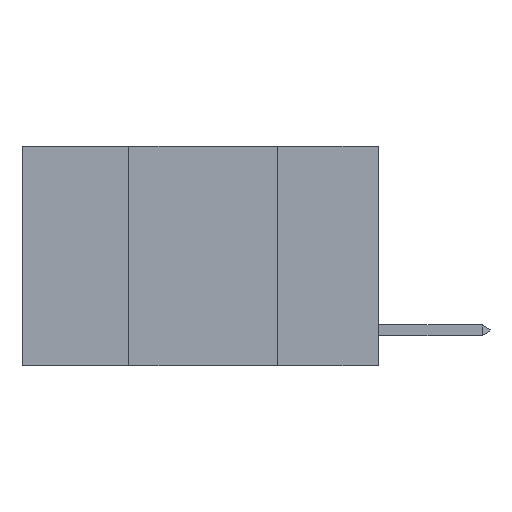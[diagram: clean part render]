
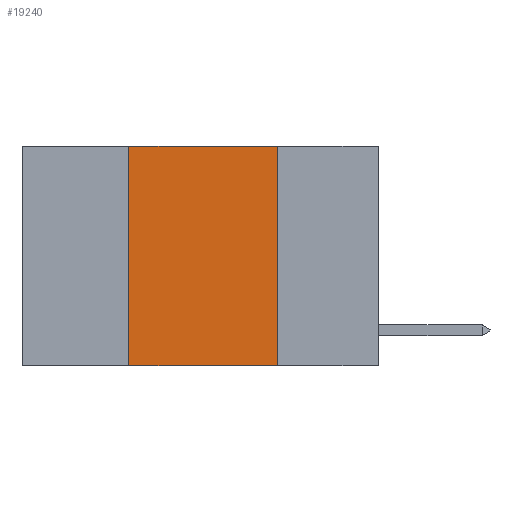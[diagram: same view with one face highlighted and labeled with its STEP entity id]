
A CAD part, left-side view. The second image highlights one B-rep face of the part: STEP entity #19240.
In plain terms, the highlighted planar face has unit normal (-1, 0, 0).
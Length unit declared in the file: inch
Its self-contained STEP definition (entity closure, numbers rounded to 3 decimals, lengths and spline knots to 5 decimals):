
#706 = EDGE_CURVE ( 'NONE', #14869, #10203, #7863, .T. ) ;
#1001 = DIRECTION ( 'NONE',  ( 0., 0., -1. ) ) ;
#1311 = EDGE_CURVE ( 'NONE', #8080, #14869, #18511, .T. ) ;
#1592 = DIRECTION ( 'NONE',  ( 0., -1., 0. ) ) ;
#1633 = FACE_OUTER_BOUND ( 'NONE', #23182, .T. ) ;
#1750 = DIRECTION ( 'NONE',  ( 1., 0., 0. ) ) ;
#4243 = VECTOR ( 'NONE', #1592, 39.37008 ) ;
#5598 = PLANE ( 'NONE',  #17433 ) ;
#6063 = VERTEX_POINT ( 'NONE', #21612 ) ;
#7863 = LINE ( 'NONE', #9908, #4243 ) ;
#8080 = VERTEX_POINT ( 'NONE', #22482 ) ;
#8596 = CARTESIAN_POINT ( 'NONE',  ( 0., 0.42, 0. ) ) ;
#8612 = VECTOR ( 'NONE', #1001, 39.37008 ) ;
#9591 = DIRECTION ( 'NONE',  ( 0., 0., -1. ) ) ;
#9908 = CARTESIAN_POINT ( 'NONE',  ( 0., 0.6, 0. ) ) ;
#10153 = CARTESIAN_POINT ( 'NONE',  ( 0., 0.6, -0.37 ) ) ;
#10203 = VERTEX_POINT ( 'NONE', #22650 ) ;
#10621 = DIRECTION ( 'NONE',  ( 0., 0., 1. ) ) ;
#12024 = ORIENTED_EDGE ( 'NONE', *, *, #1311, .F. ) ;
#12435 = VECTOR ( 'NONE', #22037, 39.37008 ) ;
#13626 = ORIENTED_EDGE ( 'NONE', *, *, #706, .F. ) ;
#14026 = CARTESIAN_POINT ( 'NONE',  ( 0., 0.42, 0. ) ) ;
#14869 = VERTEX_POINT ( 'NONE', #14026 ) ;
#16637 = ORIENTED_EDGE ( 'NONE', *, *, #16826, .T. ) ;
#16826 = EDGE_CURVE ( 'NONE', #8080, #6063, #23457, .T. ) ;
#17433 = AXIS2_PLACEMENT_3D ( 'NONE', #22872, #1750, #9591 ) ;
#18511 = LINE ( 'NONE', #8596, #21848 ) ;
#19240 = ADVANCED_FACE ( 'NONE', ( #1633 ), #5598, .F. ) ;
#20703 = CARTESIAN_POINT ( 'NONE',  ( 0., 0.17, 0. ) ) ;
#21027 = ORIENTED_EDGE ( 'NONE', *, *, #24124, .F. ) ;
#21612 = CARTESIAN_POINT ( 'NONE',  ( 0., 0.17, -0.37 ) ) ;
#21848 = VECTOR ( 'NONE', #10621, 39.37008 ) ;
#22037 = DIRECTION ( 'NONE',  ( 0., -1., 0. ) ) ;
#22482 = CARTESIAN_POINT ( 'NONE',  ( 0., 0.42, -0.37 ) ) ;
#22499 = LINE ( 'NONE', #20703, #8612 ) ;
#22650 = CARTESIAN_POINT ( 'NONE',  ( 0., 0.17, 0. ) ) ;
#22872 = CARTESIAN_POINT ( 'NONE',  ( 0., 0.6, 0. ) ) ;
#23182 = EDGE_LOOP ( 'NONE', ( #21027, #13626, #12024, #16637 ) ) ;
#23457 = LINE ( 'NONE', #10153, #12435 ) ;
#24124 = EDGE_CURVE ( 'NONE', #10203, #6063, #22499, .T. ) ;
